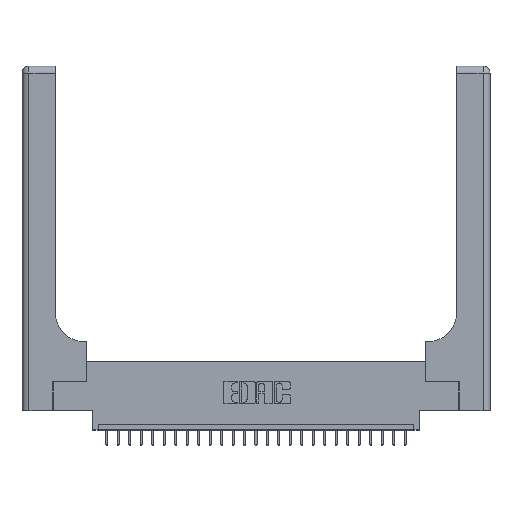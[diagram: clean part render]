
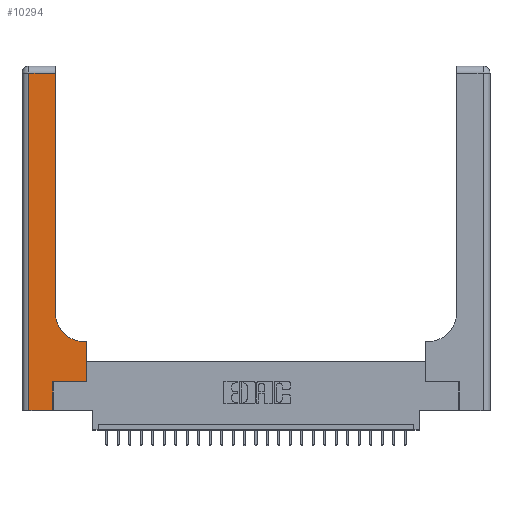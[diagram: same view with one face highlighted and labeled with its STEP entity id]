
A CAD part, top view. The second image highlights one B-rep face of the part: STEP entity #10294.
In plain terms, the highlighted planar face has unit normal (0, 0, 1).
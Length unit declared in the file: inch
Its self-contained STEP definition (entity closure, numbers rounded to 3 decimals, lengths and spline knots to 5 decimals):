
#431 = CARTESIAN_POINT ( 'NONE',  ( 0.5585, 0.6, 0.37 ) ) ;
#559 = VERTEX_POINT ( 'NONE', #12130 ) ;
#1040 = DIRECTION ( 'NONE',  ( 0., -1., 0. ) ) ;
#1255 = ORIENTED_EDGE ( 'NONE', *, *, #12371, .T. ) ;
#1926 = VERTEX_POINT ( 'NONE', #6018 ) ;
#2329 = VERTEX_POINT ( 'NONE', #26181 ) ;
#3950 = DIRECTION ( 'NONE',  ( 0., 1., 0. ) ) ;
#4018 = LINE ( 'NONE', #21183, #20103 ) ;
#4051 = ORIENTED_EDGE ( 'NONE', *, *, #18256, .T. ) ;
#4053 = CARTESIAN_POINT ( 'NONE',  ( 0.269, 0.25, 0.37 ) ) ;
#5240 = CARTESIAN_POINT ( 'NONE',  ( 0.06, 3., 0.37 ) ) ;
#5266 = ORIENTED_EDGE ( 'NONE', *, *, #18472, .T. ) ;
#5274 = LINE ( 'NONE', #13971, #15665 ) ;
#5512 = CARTESIAN_POINT ( 'NONE',  ( 0.2915, 2.94, 0.37 ) ) ;
#5686 = CARTESIAN_POINT ( 'NONE',  ( 0., 3., 0.37 ) ) ;
#6018 = CARTESIAN_POINT ( 'NONE',  ( 0.269, 0., 0.37 ) ) ;
#6253 = EDGE_CURVE ( 'NONE', #12158, #25014, #4018, .T. ) ;
#6540 = DIRECTION ( 'NONE',  ( 1., 0., 0. ) ) ;
#6786 = LINE ( 'NONE', #25857, #13931 ) ;
#7260 = VECTOR ( 'NONE', #8909, 39.37008 ) ;
#7386 = AXIS2_PLACEMENT_3D ( 'NONE', #12691, #17479, #6540 ) ;
#7630 = EDGE_CURVE ( 'NONE', #2329, #1926, #5274, .T. ) ;
#8020 = DIRECTION ( 'NONE',  ( 1., 0., 0. ) ) ;
#8823 = VECTOR ( 'NONE', #1040, 39.37008 ) ;
#8909 = DIRECTION ( 'NONE',  ( 0., 1., 0. ) ) ;
#9452 = ORIENTED_EDGE ( 'NONE', *, *, #24131, .T. ) ;
#9880 = LINE ( 'NONE', #5240, #8823 ) ;
#9967 = VECTOR ( 'NONE', #16831, 39.37008 ) ;
#10258 = EDGE_CURVE ( 'NONE', #1926, #559, #26322, .T. ) ;
#10294 = ADVANCED_FACE ( 'NONE', ( #16214 ), #27009, .F. ) ;
#10296 = ORIENTED_EDGE ( 'NONE', *, *, #11731, .T. ) ;
#10775 = LINE ( 'NONE', #25795, #9967 ) ;
#10999 = CARTESIAN_POINT ( 'NONE',  ( 0.269, 0., 0.37 ) ) ;
#11353 = VECTOR ( 'NONE', #21773, 39.37008 ) ;
#11731 = EDGE_CURVE ( 'NONE', #22930, #12158, #6786, .T. ) ;
#12130 = CARTESIAN_POINT ( 'NONE',  ( 0.269, 0.25, 0.37 ) ) ;
#12158 = VERTEX_POINT ( 'NONE', #431 ) ;
#12213 = LINE ( 'NONE', #4053, #16307 ) ;
#12315 = ORIENTED_EDGE ( 'NONE', *, *, #10258, .T. ) ;
#12371 = EDGE_CURVE ( 'NONE', #15047, #26037, #10775, .T. ) ;
#12691 = CARTESIAN_POINT ( 'NONE',  ( 0.5415, 0.85, 0.37 ) ) ;
#13522 = AXIS2_PLACEMENT_3D ( 'NONE', #5686, #24775, #20301 ) ;
#13693 = DIRECTION ( 'NONE',  ( 1., 0., 0. ) ) ;
#13834 = CARTESIAN_POINT ( 'NONE',  ( 0.06, 2.94, 0.37 ) ) ;
#13931 = VECTOR ( 'NONE', #3950, 39.37008 ) ;
#13971 = CARTESIAN_POINT ( 'NONE',  ( 0., 0., 0.37 ) ) ;
#14972 = CIRCLE ( 'NONE', #7386, 0.25 ) ;
#14994 = CARTESIAN_POINT ( 'NONE',  ( 0.2915, 0.85, 0.37 ) ) ;
#15047 = VERTEX_POINT ( 'NONE', #5512 ) ;
#15665 = VECTOR ( 'NONE', #13693, 39.37008 ) ;
#16087 = EDGE_CURVE ( 'NONE', #25014, #18384, #14972, .T. ) ;
#16214 = FACE_OUTER_BOUND ( 'NONE', #16218, .T. ) ;
#16218 = EDGE_LOOP ( 'NONE', ( #5266, #1255, #9452, #23550, #12315, #4051, #10296, #23478, #22740 ) ) ;
#16307 = VECTOR ( 'NONE', #8020, 39.37008 ) ;
#16831 = DIRECTION ( 'NONE',  ( -1., 0., 0. ) ) ;
#16953 = DIRECTION ( 'NONE',  ( -1., 0., 0. ) ) ;
#17263 = CARTESIAN_POINT ( 'NONE',  ( 0.2915, 3., 0.37 ) ) ;
#17479 = DIRECTION ( 'NONE',  ( 0., 0., -1. ) ) ;
#18256 = EDGE_CURVE ( 'NONE', #559, #22930, #12213, .T. ) ;
#18384 = VERTEX_POINT ( 'NONE', #14994 ) ;
#18472 = EDGE_CURVE ( 'NONE', #18384, #15047, #19813, .T. ) ;
#18723 = CARTESIAN_POINT ( 'NONE',  ( 0.5585, 0.25, 0.37 ) ) ;
#19813 = LINE ( 'NONE', #17263, #11353 ) ;
#20103 = VECTOR ( 'NONE', #16953, 39.37008 ) ;
#20301 = DIRECTION ( 'NONE',  ( -1., 0., 0. ) ) ;
#21183 = CARTESIAN_POINT ( 'NONE',  ( 0.2915, 0.6, 0.37 ) ) ;
#21773 = DIRECTION ( 'NONE',  ( 0., 1., 0. ) ) ;
#22740 = ORIENTED_EDGE ( 'NONE', *, *, #16087, .T. ) ;
#22930 = VERTEX_POINT ( 'NONE', #18723 ) ;
#23478 = ORIENTED_EDGE ( 'NONE', *, *, #6253, .T. ) ;
#23550 = ORIENTED_EDGE ( 'NONE', *, *, #7630, .T. ) ;
#24131 = EDGE_CURVE ( 'NONE', #26037, #2329, #9880, .T. ) ;
#24775 = DIRECTION ( 'NONE',  ( 0., 0., -1. ) ) ;
#25014 = VERTEX_POINT ( 'NONE', #25239 ) ;
#25239 = CARTESIAN_POINT ( 'NONE',  ( 0.5415, 0.6, 0.37 ) ) ;
#25795 = CARTESIAN_POINT ( 'NONE',  ( 0., 2.94, 0.37 ) ) ;
#25857 = CARTESIAN_POINT ( 'NONE',  ( 0.5585, 0.25, 0.37 ) ) ;
#26037 = VERTEX_POINT ( 'NONE', #13834 ) ;
#26181 = CARTESIAN_POINT ( 'NONE',  ( 0.06, 0., 0.37 ) ) ;
#26322 = LINE ( 'NONE', #10999, #7260 ) ;
#27009 = PLANE ( 'NONE',  #13522 ) ;
